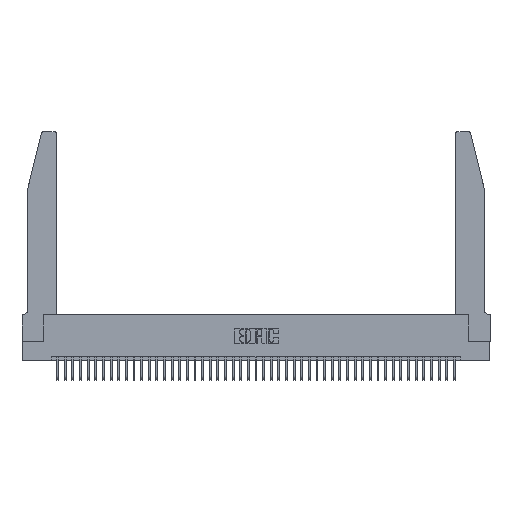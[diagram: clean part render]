
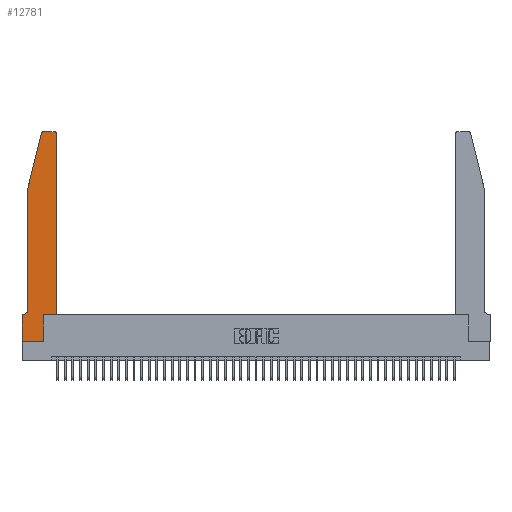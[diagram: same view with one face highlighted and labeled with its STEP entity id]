
A CAD part, top view. The second image highlights one B-rep face of the part: STEP entity #12781.
In plain terms, the highlighted planar face has unit normal (0, 0, 1).
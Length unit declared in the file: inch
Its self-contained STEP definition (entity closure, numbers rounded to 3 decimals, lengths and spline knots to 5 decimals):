
#370 = CIRCLE ( 'NONE', #17707, 0.07 ) ;
#903 = EDGE_CURVE ( 'NONE', #31453, #22971, #26668, .T. ) ;
#1109 = DIRECTION ( 'NONE',  ( 1., 0., 0. ) ) ;
#1660 = LINE ( 'NONE', #40617, #17338 ) ;
#1846 = VERTEX_POINT ( 'NONE', #23153 ) ;
#2632 = EDGE_CURVE ( 'NONE', #3334, #29307, #23426, .T. ) ;
#2688 = CARTESIAN_POINT ( 'NONE',  ( 0.4205, 2.72, 0.37 ) ) ;
#2776 = CARTESIAN_POINT ( 'NONE',  ( 0.2865, 0., 0.37 ) ) ;
#3273 = VECTOR ( 'NONE', #6019, 39.37008 ) ;
#3334 = VERTEX_POINT ( 'NONE', #14003 ) ;
#3375 = VERTEX_POINT ( 'NONE', #34343 ) ;
#3504 = CARTESIAN_POINT ( 'NONE',  ( 0.2865, 0.35, 0.37 ) ) ;
#4943 = VERTEX_POINT ( 'NONE', #3504 ) ;
#5733 = VERTEX_POINT ( 'NONE', #30927 ) ;
#6019 = DIRECTION ( 'NONE',  ( 1., 0., 0. ) ) ;
#6062 = DIRECTION ( 'NONE',  ( 1., 0., 0. ) ) ;
#6136 = VECTOR ( 'NONE', #41826, 39.37008 ) ;
#7047 = CARTESIAN_POINT ( 'NONE',  ( 0.0755, 2., 0.37 ) ) ;
#7352 = DIRECTION ( 'NONE',  ( 1., 0., 0. ) ) ;
#7535 = CARTESIAN_POINT ( 'NONE',  ( 0.2865, 0.35, 0.37 ) ) ;
#9581 = EDGE_CURVE ( 'NONE', #31451, #31453, #40577, .T. ) ;
#9788 = VECTOR ( 'NONE', #26125, 39.37008 ) ;
#10401 = VERTEX_POINT ( 'NONE', #17034 ) ;
#10405 = DIRECTION ( 'NONE',  ( 0., 0., 1. ) ) ;
#12781 = ADVANCED_FACE ( 'NONE', ( #29928 ), #27055, .T. ) ;
#13032 = CARTESIAN_POINT ( 'NONE',  ( 0.0055, 0.42, 0.37 ) ) ;
#13639 = EDGE_CURVE ( 'NONE', #10401, #3334, #23755, .T. ) ;
#14003 = CARTESIAN_POINT ( 'NONE',  ( 0.4205, 2.75, 0.37 ) ) ;
#14364 = DIRECTION ( 'NONE',  ( -1., 0., 0. ) ) ;
#14647 = CARTESIAN_POINT ( 'NONE',  ( 0.0755, 2., 0.37 ) ) ;
#14800 = ORIENTED_EDGE ( 'NONE', *, *, #30881, .T. ) ;
#15079 = AXIS2_PLACEMENT_3D ( 'NONE', #41124, #21138, #1109 ) ;
#15719 = ORIENTED_EDGE ( 'NONE', *, *, #903, .T. ) ;
#15734 = EDGE_CURVE ( 'NONE', #4943, #3375, #1660, .T. ) ;
#16062 = CARTESIAN_POINT ( 'NONE',  ( 0.4505, 0.35, 0.37 ) ) ;
#16387 = DIRECTION ( 'NONE',  ( -1., 0., 0. ) ) ;
#16616 = VECTOR ( 'NONE', #14364, 39.37008 ) ;
#17034 = CARTESIAN_POINT ( 'NONE',  ( 0.4505, 2.72, 0.37 ) ) ;
#17338 = VECTOR ( 'NONE', #7352, 39.37008 ) ;
#17707 = AXIS2_PLACEMENT_3D ( 'NONE', #13032, #36438, #16387 ) ;
#18404 = DIRECTION ( 'NONE',  ( 0., -1., 0. ) ) ;
#18690 = LINE ( 'NONE', #40899, #16616 ) ;
#18924 = ORIENTED_EDGE ( 'NONE', *, *, #23885, .T. ) ;
#19708 = LINE ( 'NONE', #16062, #9788 ) ;
#20188 = VECTOR ( 'NONE', #27521, 39.37008 ) ;
#20446 = DIRECTION ( 'NONE',  ( -1., 0., 0. ) ) ;
#21138 = DIRECTION ( 'NONE',  ( 0., 0., 1. ) ) ;
#21269 = LINE ( 'NONE', #7535, #20188 ) ;
#22376 = VECTOR ( 'NONE', #20446, 39.37008 ) ;
#22483 = VECTOR ( 'NONE', #18404, 39.37008 ) ;
#22647 = CARTESIAN_POINT ( 'NONE',  ( 0., 0., 0.37 ) ) ;
#22971 = VERTEX_POINT ( 'NONE', #24905 ) ;
#23153 = CARTESIAN_POINT ( 'NONE',  ( 0.0055, 0.35, 0.37 ) ) ;
#23426 = LINE ( 'NONE', #23689, #22376 ) ;
#23498 = EDGE_CURVE ( 'NONE', #1846, #5733, #18690, .T. ) ;
#23689 = CARTESIAN_POINT ( 'NONE',  ( 0.2605, 2.75, 0.37 ) ) ;
#23755 = CIRCLE ( 'NONE', #40694, 0.03 ) ;
#23885 = EDGE_CURVE ( 'NONE', #3375, #10401, #19708, .T. ) ;
#23918 = VERTEX_POINT ( 'NONE', #2776 ) ;
#24905 = CARTESIAN_POINT ( 'NONE',  ( 0.0755, 0.42, 0.37 ) ) ;
#25442 = EDGE_LOOP ( 'NONE', ( #30082, #35836, #40329, #15719, #29328, #31929, #32315, #32621, #14800, #29258, #18924, #26454 ) ) ;
#26038 = DIRECTION ( 'NONE',  ( 0., 0., 1. ) ) ;
#26125 = DIRECTION ( 'NONE',  ( 0., 1., 0. ) ) ;
#26454 = ORIENTED_EDGE ( 'NONE', *, *, #13639, .T. ) ;
#26668 = LINE ( 'NONE', #41624, #22483 ) ;
#27026 = CARTESIAN_POINT ( 'NONE',  ( 0.25487, 2.72718, 0.37 ) ) ;
#27055 = PLANE ( 'NONE',  #33487 ) ;
#27484 = VERTEX_POINT ( 'NONE', #36518 ) ;
#27521 = DIRECTION ( 'NONE',  ( 0., 1., 0. ) ) ;
#29258 = ORIENTED_EDGE ( 'NONE', *, *, #15734, .T. ) ;
#29307 = VERTEX_POINT ( 'NONE', #39618 ) ;
#29328 = ORIENTED_EDGE ( 'NONE', *, *, #33208, .T. ) ;
#29928 = FACE_OUTER_BOUND ( 'NONE', #25442, .T. ) ;
#29952 = LINE ( 'NONE', #22647, #3273 ) ;
#30082 = ORIENTED_EDGE ( 'NONE', *, *, #2632, .T. ) ;
#30475 = CARTESIAN_POINT ( 'NONE',  ( 0., 0.35, 0.37 ) ) ;
#30881 = EDGE_CURVE ( 'NONE', #23918, #4943, #21269, .T. ) ;
#30927 = CARTESIAN_POINT ( 'NONE',  ( 0., 0.35, 0.37 ) ) ;
#31451 = VERTEX_POINT ( 'NONE', #27026 ) ;
#31453 = VERTEX_POINT ( 'NONE', #7047 ) ;
#31929 = ORIENTED_EDGE ( 'NONE', *, *, #23498, .T. ) ;
#32315 = ORIENTED_EDGE ( 'NONE', *, *, #41009, .T. ) ;
#32621 = ORIENTED_EDGE ( 'NONE', *, *, #36844, .T. ) ;
#32836 = LINE ( 'NONE', #38521, #6136 ) ;
#33208 = EDGE_CURVE ( 'NONE', #22971, #1846, #370, .T. ) ;
#33487 = AXIS2_PLACEMENT_3D ( 'NONE', #30475, #10405, #33844 ) ;
#33844 = DIRECTION ( 'NONE',  ( 1., 0., 0. ) ) ;
#34343 = CARTESIAN_POINT ( 'NONE',  ( 0.4505, 0.35, 0.37 ) ) ;
#35836 = ORIENTED_EDGE ( 'NONE', *, *, #40855, .T. ) ;
#36438 = DIRECTION ( 'NONE',  ( 0., 0., -1. ) ) ;
#36518 = CARTESIAN_POINT ( 'NONE',  ( 0., 0., 0.37 ) ) ;
#36844 = EDGE_CURVE ( 'NONE', #27484, #23918, #29952, .T. ) ;
#38037 = DIRECTION ( 'NONE',  ( -0.239, -0.971, 0. ) ) ;
#38521 = CARTESIAN_POINT ( 'NONE',  ( 0., 0., 0.37 ) ) ;
#39618 = CARTESIAN_POINT ( 'NONE',  ( 0.284, 2.75, 0.37 ) ) ;
#40110 = CIRCLE ( 'NONE', #15079, 0.03 ) ;
#40329 = ORIENTED_EDGE ( 'NONE', *, *, #9581, .T. ) ;
#40577 = LINE ( 'NONE', #14647, #41617 ) ;
#40617 = CARTESIAN_POINT ( 'NONE',  ( 0.4505, 0.35, 0.37 ) ) ;
#40694 = AXIS2_PLACEMENT_3D ( 'NONE', #2688, #26038, #6062 ) ;
#40855 = EDGE_CURVE ( 'NONE', #29307, #31451, #40110, .T. ) ;
#40899 = CARTESIAN_POINT ( 'NONE',  ( 0.0755, 0.35, 0.37 ) ) ;
#41009 = EDGE_CURVE ( 'NONE', #5733, #27484, #32836, .T. ) ;
#41124 = CARTESIAN_POINT ( 'NONE',  ( 0.284, 2.72, 0.37 ) ) ;
#41617 = VECTOR ( 'NONE', #38037, 39.37008 ) ;
#41624 = CARTESIAN_POINT ( 'NONE',  ( 0.0755, 2., 0.37 ) ) ;
#41826 = DIRECTION ( 'NONE',  ( 0., -1., 0. ) ) ;
